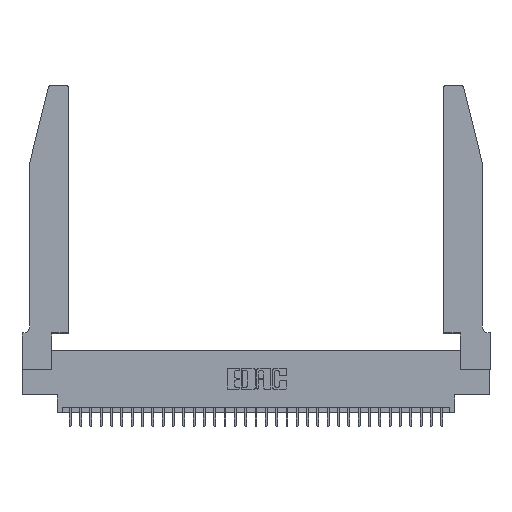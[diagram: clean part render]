
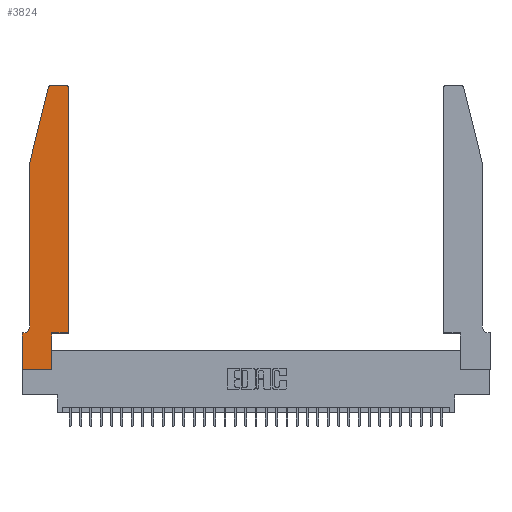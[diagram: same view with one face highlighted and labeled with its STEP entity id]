
A CAD part, top view. The second image highlights one B-rep face of the part: STEP entity #3824.
In plain terms, the highlighted planar face has unit normal (0, 0, 1).
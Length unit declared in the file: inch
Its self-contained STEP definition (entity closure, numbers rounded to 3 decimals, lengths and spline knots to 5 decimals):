
#304 = VERTEX_POINT ( 'NONE', #26512 ) ;
#472 = CARTESIAN_POINT ( 'NONE',  ( 0.2865, 0., 0.37 ) ) ;
#548 = CARTESIAN_POINT ( 'NONE',  ( 0.4505, 0.35, 0.37 ) ) ;
#567 = DIRECTION ( 'NONE',  ( -1., 0., 0. ) ) ;
#1271 = DIRECTION ( 'NONE',  ( 0., 0., 1. ) ) ;
#1452 = CARTESIAN_POINT ( 'NONE',  ( 0.284, 2.72, 0.37 ) ) ;
#2172 = DIRECTION ( 'NONE',  ( -1., 0., 0. ) ) ;
#2795 = VECTOR ( 'NONE', #5370, 39.37008 ) ;
#3363 = CARTESIAN_POINT ( 'NONE',  ( 0.4205, 2.75, 0.37 ) ) ;
#3545 = DIRECTION ( 'NONE',  ( 1., 0., 0. ) ) ;
#3824 = ADVANCED_FACE ( 'NONE', ( #22258 ), #22766, .T. ) ;
#3893 = ORIENTED_EDGE ( 'NONE', *, *, #10501, .T. ) ;
#3982 = DIRECTION ( 'NONE',  ( 1., 0., 0. ) ) ;
#3988 = EDGE_CURVE ( 'NONE', #4564, #19694, #21528, .T. ) ;
#4467 = AXIS2_PLACEMENT_3D ( 'NONE', #29549, #31828, #5654 ) ;
#4499 = VECTOR ( 'NONE', #33756, 39.37008 ) ;
#4564 = VERTEX_POINT ( 'NONE', #23277 ) ;
#5326 = ORIENTED_EDGE ( 'NONE', *, *, #11411, .T. ) ;
#5370 = DIRECTION ( 'NONE',  ( 1., 0., 0. ) ) ;
#5654 = DIRECTION ( 'NONE',  ( 1., 0., 0. ) ) ;
#6229 = VERTEX_POINT ( 'NONE', #21165 ) ;
#6290 = CARTESIAN_POINT ( 'NONE',  ( 0., 0.35, 0.37 ) ) ;
#7057 = VERTEX_POINT ( 'NONE', #3363 ) ;
#7127 = EDGE_CURVE ( 'NONE', #10091, #15975, #27591, .T. ) ;
#7809 = AXIS2_PLACEMENT_3D ( 'NONE', #6290, #8542, #3982 ) ;
#8200 = CARTESIAN_POINT ( 'NONE',  ( 0., 0.35, 0.37 ) ) ;
#8517 = VECTOR ( 'NONE', #3545, 39.37008 ) ;
#8528 = AXIS2_PLACEMENT_3D ( 'NONE', #14762, #24787, #32892 ) ;
#8542 = DIRECTION ( 'NONE',  ( 0., 0., 1. ) ) ;
#8631 = EDGE_CURVE ( 'NONE', #26066, #32638, #12886, .T. ) ;
#9154 = LINE ( 'NONE', #11968, #4499 ) ;
#9470 = VECTOR ( 'NONE', #2172, 39.37008 ) ;
#10091 = VERTEX_POINT ( 'NONE', #11966 ) ;
#10171 = LINE ( 'NONE', #23346, #13302 ) ;
#10501 = EDGE_CURVE ( 'NONE', #19694, #16025, #31531, .T. ) ;
#10566 = CARTESIAN_POINT ( 'NONE',  ( 0.0755, 0.35, 0.37 ) ) ;
#10878 = LINE ( 'NONE', #13193, #20104 ) ;
#10923 = CARTESIAN_POINT ( 'NONE',  ( 0.2605, 2.75, 0.37 ) ) ;
#11411 = EDGE_CURVE ( 'NONE', #6229, #28719, #10171, .T. ) ;
#11966 = CARTESIAN_POINT ( 'NONE',  ( 0., 0., 0.37 ) ) ;
#11968 = CARTESIAN_POINT ( 'NONE',  ( 0.2865, 0.35, 0.37 ) ) ;
#12214 = ORIENTED_EDGE ( 'NONE', *, *, #8631, .T. ) ;
#12256 = ORIENTED_EDGE ( 'NONE', *, *, #33411, .T. ) ;
#12886 = LINE ( 'NONE', #10566, #9470 ) ;
#12923 = EDGE_CURVE ( 'NONE', #28719, #18309, #10878, .T. ) ;
#13193 = CARTESIAN_POINT ( 'NONE',  ( 0.0755, 2., 0.37 ) ) ;
#13262 = ORIENTED_EDGE ( 'NONE', *, *, #29179, .T. ) ;
#13278 = CARTESIAN_POINT ( 'NONE',  ( 0.4505, 0.35, 0.37 ) ) ;
#13302 = VECTOR ( 'NONE', #18265, 39.37008 ) ;
#13541 = DIRECTION ( 'NONE',  ( 0., -1., 0. ) ) ;
#14088 = DIRECTION ( 'NONE',  ( 0., -1., 0. ) ) ;
#14399 = CIRCLE ( 'NONE', #29531, 0.03 ) ;
#14762 = CARTESIAN_POINT ( 'NONE',  ( 0.0055, 0.42, 0.37 ) ) ;
#15054 = EDGE_LOOP ( 'NONE', ( #15754, #21212, #5326, #16630, #12256, #12214, #15996, #26679, #13262, #23974, #3893, #20766 ) ) ;
#15055 = EDGE_CURVE ( 'NONE', #16025, #7057, #15667, .T. ) ;
#15537 = CARTESIAN_POINT ( 'NONE',  ( 0.4505, 0.35, 0.37 ) ) ;
#15667 = CIRCLE ( 'NONE', #4467, 0.03 ) ;
#15754 = ORIENTED_EDGE ( 'NONE', *, *, #29131, .T. ) ;
#15975 = VERTEX_POINT ( 'NONE', #472 ) ;
#15996 = ORIENTED_EDGE ( 'NONE', *, *, #21941, .T. ) ;
#16025 = VERTEX_POINT ( 'NONE', #27688 ) ;
#16180 = LINE ( 'NONE', #27227, #31652 ) ;
#16630 = ORIENTED_EDGE ( 'NONE', *, *, #12923, .T. ) ;
#17511 = CARTESIAN_POINT ( 'NONE',  ( 0.0755, 2., 0.37 ) ) ;
#18253 = DIRECTION ( 'NONE',  ( 1., 0., 0. ) ) ;
#18265 = DIRECTION ( 'NONE',  ( -0.239, -0.971, 0. ) ) ;
#18309 = VERTEX_POINT ( 'NONE', #30816 ) ;
#19022 = LINE ( 'NONE', #10923, #21315 ) ;
#19694 = VERTEX_POINT ( 'NONE', #548 ) ;
#20104 = VECTOR ( 'NONE', #13541, 39.37008 ) ;
#20766 = ORIENTED_EDGE ( 'NONE', *, *, #15055, .T. ) ;
#21165 = CARTESIAN_POINT ( 'NONE',  ( 0.25487, 2.72718, 0.37 ) ) ;
#21212 = ORIENTED_EDGE ( 'NONE', *, *, #24527, .T. ) ;
#21315 = VECTOR ( 'NONE', #567, 39.37008 ) ;
#21528 = LINE ( 'NONE', #13278, #2795 ) ;
#21941 = EDGE_CURVE ( 'NONE', #32638, #10091, #16180, .T. ) ;
#22258 = FACE_OUTER_BOUND ( 'NONE', #15054, .T. ) ;
#22766 = PLANE ( 'NONE',  #7809 ) ;
#23277 = CARTESIAN_POINT ( 'NONE',  ( 0.2865, 0.35, 0.37 ) ) ;
#23346 = CARTESIAN_POINT ( 'NONE',  ( 0.0755, 2., 0.37 ) ) ;
#23974 = ORIENTED_EDGE ( 'NONE', *, *, #3988, .T. ) ;
#24527 = EDGE_CURVE ( 'NONE', #304, #6229, #14399, .T. ) ;
#24787 = DIRECTION ( 'NONE',  ( 0., 0., -1. ) ) ;
#26066 = VERTEX_POINT ( 'NONE', #29291 ) ;
#26512 = CARTESIAN_POINT ( 'NONE',  ( 0.284, 2.75, 0.37 ) ) ;
#26679 = ORIENTED_EDGE ( 'NONE', *, *, #7127, .T. ) ;
#27227 = CARTESIAN_POINT ( 'NONE',  ( 0., 0., 0.37 ) ) ;
#27591 = LINE ( 'NONE', #33398, #8517 ) ;
#27688 = CARTESIAN_POINT ( 'NONE',  ( 0.4505, 2.72, 0.37 ) ) ;
#28719 = VERTEX_POINT ( 'NONE', #17511 ) ;
#29131 = EDGE_CURVE ( 'NONE', #7057, #304, #19022, .T. ) ;
#29179 = EDGE_CURVE ( 'NONE', #15975, #4564, #9154, .T. ) ;
#29291 = CARTESIAN_POINT ( 'NONE',  ( 0.0055, 0.35, 0.37 ) ) ;
#29531 = AXIS2_PLACEMENT_3D ( 'NONE', #1452, #1271, #18253 ) ;
#29549 = CARTESIAN_POINT ( 'NONE',  ( 0.4205, 2.72, 0.37 ) ) ;
#30816 = CARTESIAN_POINT ( 'NONE',  ( 0.0755, 0.42, 0.37 ) ) ;
#31531 = LINE ( 'NONE', #15537, #34549 ) ;
#31548 = CIRCLE ( 'NONE', #8528, 0.07 ) ;
#31652 = VECTOR ( 'NONE', #14088, 39.37008 ) ;
#31828 = DIRECTION ( 'NONE',  ( 0., 0., 1. ) ) ;
#31867 = DIRECTION ( 'NONE',  ( 0., 1., 0. ) ) ;
#32638 = VERTEX_POINT ( 'NONE', #8200 ) ;
#32892 = DIRECTION ( 'NONE',  ( -1., 0., 0. ) ) ;
#33398 = CARTESIAN_POINT ( 'NONE',  ( 0., 0., 0.37 ) ) ;
#33411 = EDGE_CURVE ( 'NONE', #18309, #26066, #31548, .T. ) ;
#33756 = DIRECTION ( 'NONE',  ( 0., 1., 0. ) ) ;
#34549 = VECTOR ( 'NONE', #31867, 39.37008 ) ;
